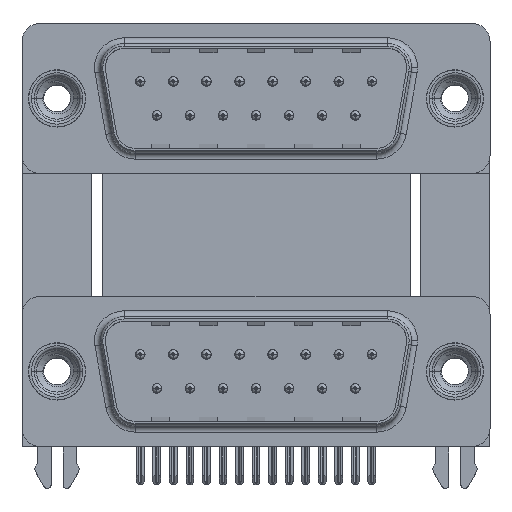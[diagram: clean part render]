
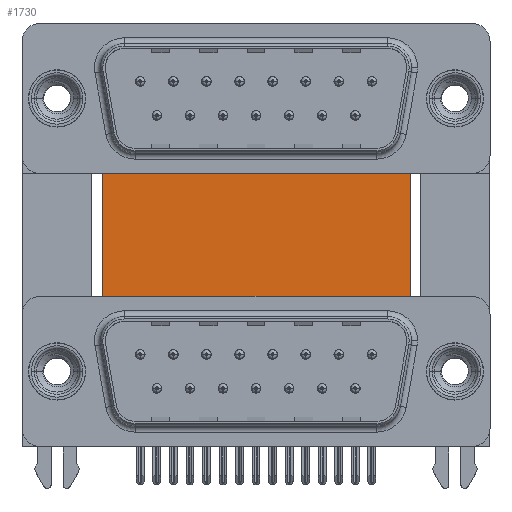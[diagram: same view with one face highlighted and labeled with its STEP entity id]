
A CAD part, top view. The second image highlights one B-rep face of the part: STEP entity #1730.
In plain terms, the highlighted planar face has unit normal (0, 0, 1).
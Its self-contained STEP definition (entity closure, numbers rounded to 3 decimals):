
#413 = DIRECTION ( 'NONE',  ( 1., 0., 0. ) ) ;
#506 = EDGE_CURVE ( 'NONE', #19190, #17574, #25988, .T. ) ;
#1588 = DIRECTION ( 'NONE',  ( 0., -1., 0. ) ) ;
#1730 = ADVANCED_FACE ( 'NONE', ( #16951 ), #32245, .F. ) ;
#1913 = CARTESIAN_POINT ( 'NONE',  ( 3.79, 16.585, -12. ) ) ;
#2790 = LINE ( 'NONE', #5707, #4255 ) ;
#3400 = VERTEX_POINT ( 'NONE', #29151 ) ;
#3501 = CARTESIAN_POINT ( 'NONE',  ( 3.79, 16.585, -12. ) ) ;
#3558 = CARTESIAN_POINT ( 'NONE',  ( 29.58, -3.735, -12. ) ) ;
#4255 = VECTOR ( 'NONE', #21712, 1000. ) ;
#4322 = ORIENTED_EDGE ( 'NONE', *, *, #20276, .T. ) ;
#5707 = CARTESIAN_POINT ( 'NONE',  ( 3.79, -3.735, -12. ) ) ;
#8669 = LINE ( 'NONE', #3501, #25511 ) ;
#8701 = CARTESIAN_POINT ( 'NONE',  ( 3.79, 16.585, -12. ) ) ;
#12621 = VERTEX_POINT ( 'NONE', #25299 ) ;
#13859 = VECTOR ( 'NONE', #1588, 1000. ) ;
#14646 = LINE ( 'NONE', #1913, #13859 ) ;
#14708 = EDGE_CURVE ( 'NONE', #3400, #19190, #8669, .T. ) ;
#15843 = CARTESIAN_POINT ( 'NONE',  ( 29.58, 16.585, -12. ) ) ;
#16951 = FACE_OUTER_BOUND ( 'NONE', #28531, .T. ) ;
#17574 = VERTEX_POINT ( 'NONE', #3558 ) ;
#19190 = VERTEX_POINT ( 'NONE', #23524 ) ;
#19859 = AXIS2_PLACEMENT_3D ( 'NONE', #8701, #29676, #27096 ) ;
#20276 = EDGE_CURVE ( 'NONE', #12621, #17574, #2790, .T. ) ;
#21712 = DIRECTION ( 'NONE',  ( 1., 0., 0. ) ) ;
#23524 = CARTESIAN_POINT ( 'NONE',  ( 29.58, 16.585, -12. ) ) ;
#25299 = CARTESIAN_POINT ( 'NONE',  ( 3.79, -3.735, -12. ) ) ;
#25511 = VECTOR ( 'NONE', #413, 1000. ) ;
#25988 = LINE ( 'NONE', #15843, #26875 ) ;
#26875 = VECTOR ( 'NONE', #30808, 1000. ) ;
#27096 = DIRECTION ( 'NONE',  ( -1., 0., 0. ) ) ;
#28531 = EDGE_LOOP ( 'NONE', ( #4322, #29700, #28797, #32096 ) ) ;
#28797 = ORIENTED_EDGE ( 'NONE', *, *, #14708, .F. ) ;
#28836 = EDGE_CURVE ( 'NONE', #3400, #12621, #14646, .T. ) ;
#29151 = CARTESIAN_POINT ( 'NONE',  ( 3.79, 16.585, -12. ) ) ;
#29676 = DIRECTION ( 'NONE',  ( 0., 0., -1. ) ) ;
#29700 = ORIENTED_EDGE ( 'NONE', *, *, #506, .F. ) ;
#30808 = DIRECTION ( 'NONE',  ( 0., -1., 0. ) ) ;
#32096 = ORIENTED_EDGE ( 'NONE', *, *, #28836, .T. ) ;
#32245 = PLANE ( 'NONE',  #19859 ) ;
